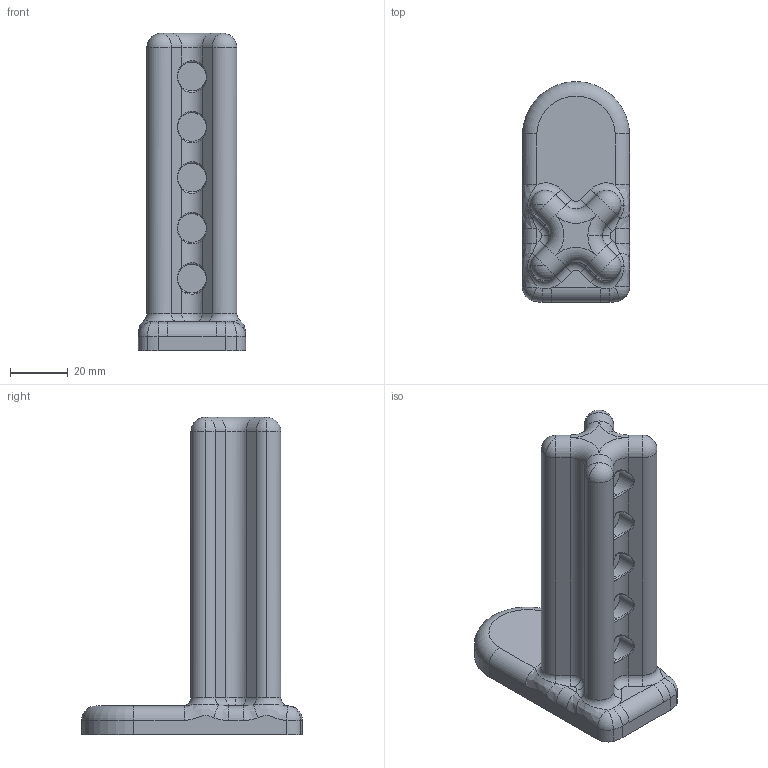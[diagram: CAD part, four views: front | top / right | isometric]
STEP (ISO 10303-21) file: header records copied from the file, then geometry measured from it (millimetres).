
FILE_DESCRIPTION (( 'STEP AP214' ), '1' );
FILE_NAME ('Stock_Arm.STEP', '2013-09-01T16:39:43', ( 'Asher' ), ( '' ), 'SwSTEP 2.0', 'SolidWorks 2013', '' );
FILE_SCHEMA (( 'AUTOMOTIVE_DESIGN' ));
Length unit declared in the file: millimetre
Products named in the file (1): Stock_Arm
Bounding box: 37.13 x 76.47 x 110 mm (x, y, z)
Volume: 90549.1 mm3; surface area: 21091.3 mm2
Topology: 1 solids, 1 shells, 147 faces, 355 edges, 208 vertices
Faces by surface type: cylinder 53, bspline 44, plane 24, torus 18, sphere 8
Entity records: 6220 total; most frequent: CARTESIAN_POINT 3108, ORIENTED_EDGE 694, DIRECTION 609, EDGE_CURVE 347, AXIS2_PLACEMENT_3D 260, VERTEX_POINT 204, CIRCLE 156, EDGE_LOOP 149
